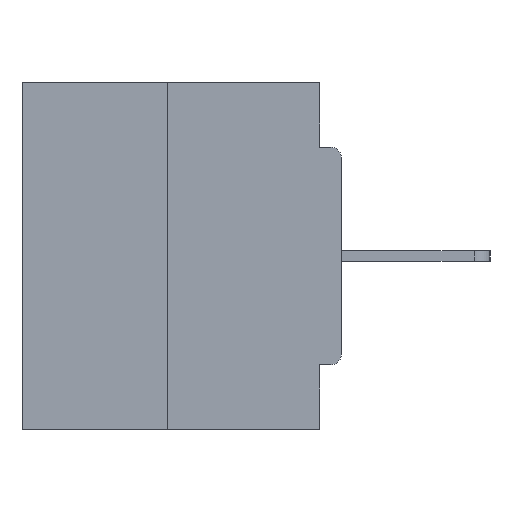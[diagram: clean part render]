
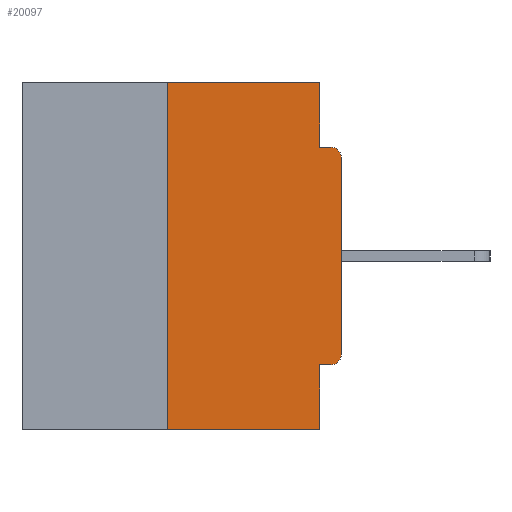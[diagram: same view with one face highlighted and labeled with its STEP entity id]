
A CAD part, left-side view. The second image highlights one B-rep face of the part: STEP entity #20097.
In plain terms, the highlighted planar face has unit normal (-1, 0, 0).
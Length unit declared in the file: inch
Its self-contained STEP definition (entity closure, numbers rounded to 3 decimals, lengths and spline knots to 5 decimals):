
#342 = VECTOR ( 'NONE', #13717, 39.37008 ) ;
#380 = DIRECTION ( 'NONE',  ( 0., 0., 1. ) ) ;
#614 = EDGE_CURVE ( 'NONE', #27230, #2154, #13152, .T. ) ;
#661 = PLANE ( 'NONE',  #5193 ) ;
#723 = AXIS2_PLACEMENT_3D ( 'NONE', #12065, #17318, #14933 ) ;
#757 = ORIENTED_EDGE ( 'NONE', *, *, #18903, .F. ) ;
#862 = ORIENTED_EDGE ( 'NONE', *, *, #25613, .F. ) ;
#1022 = CARTESIAN_POINT ( 'NONE',  ( 0., 0., -0.3915 ) ) ;
#2154 = VERTEX_POINT ( 'NONE', #19680 ) ;
#2256 = DIRECTION ( 'NONE',  ( 0., 0., -1. ) ) ;
#2449 = CARTESIAN_POINT ( 'NONE',  ( 0., 0.46, 0. ) ) ;
#2577 = CARTESIAN_POINT ( 'NONE',  ( 0., 0., 0. ) ) ;
#2992 = DIRECTION ( 'NONE',  ( 0., 0., 1. ) ) ;
#3128 = EDGE_CURVE ( 'NONE', #22360, #9366, #9825, .T. ) ;
#3137 = LINE ( 'NONE', #5524, #28542 ) ;
#3690 = ORIENTED_EDGE ( 'NONE', *, *, #25603, .F. ) ;
#3891 = EDGE_CURVE ( 'NONE', #9366, #13683, #4969, .T. ) ;
#4315 = LINE ( 'NONE', #24075, #11857 ) ;
#4780 = ORIENTED_EDGE ( 'NONE', *, *, #3891, .T. ) ;
#4822 = DIRECTION ( 'NONE',  ( 0., -1., 0. ) ) ;
#4969 = LINE ( 'NONE', #2577, #5308 ) ;
#5193 = AXIS2_PLACEMENT_3D ( 'NONE', #26952, #27274, #24726 ) ;
#5206 = CARTESIAN_POINT ( 'NONE',  ( 0., 0., -0.4065 ) ) ;
#5308 = VECTOR ( 'NONE', #380, 39.37008 ) ;
#5524 = CARTESIAN_POINT ( 'NONE',  ( 0., 0.25, 0. ) ) ;
#6390 = LINE ( 'NONE', #11798, #342 ) ;
#6964 = VERTEX_POINT ( 'NONE', #23285 ) ;
#7230 = VECTOR ( 'NONE', #17772, 39.37008 ) ;
#7241 = CARTESIAN_POINT ( 'NONE',  ( 0., 0., -0.1085 ) ) ;
#8156 = ORIENTED_EDGE ( 'NONE', *, *, #26112, .F. ) ;
#9366 = VERTEX_POINT ( 'NONE', #1022 ) ;
#9825 = CIRCLE ( 'NONE', #25092, 0.015 ) ;
#9902 = EDGE_CURVE ( 'NONE', #17924, #12149, #4315, .T. ) ;
#10376 = CIRCLE ( 'NONE', #723, 0.015 ) ;
#11001 = CARTESIAN_POINT ( 'NONE',  ( 0., 0.015, -0.4065 ) ) ;
#11742 = ORIENTED_EDGE ( 'NONE', *, *, #9902, .F. ) ;
#11798 = CARTESIAN_POINT ( 'NONE',  ( 0., 0.46, -0.5 ) ) ;
#11857 = VECTOR ( 'NONE', #2256, 39.37008 ) ;
#12065 = CARTESIAN_POINT ( 'NONE',  ( 0., 0.015, -0.1085 ) ) ;
#12149 = VERTEX_POINT ( 'NONE', #27022 ) ;
#13152 = LINE ( 'NONE', #30043, #7230 ) ;
#13683 = VERTEX_POINT ( 'NONE', #7241 ) ;
#13717 = DIRECTION ( 'NONE',  ( 0., -1., 0. ) ) ;
#14562 = LINE ( 'NONE', #26670, #14572 ) ;
#14572 = VECTOR ( 'NONE', #4822, 39.37008 ) ;
#14933 = DIRECTION ( 'NONE',  ( 0., 0., -1. ) ) ;
#15132 = DIRECTION ( 'NONE',  ( 0., 0., -1. ) ) ;
#16623 = VECTOR ( 'NONE', #17830, 39.37008 ) ;
#17158 = CARTESIAN_POINT ( 'NONE',  ( 0., 0.25, 0. ) ) ;
#17318 = DIRECTION ( 'NONE',  ( -1., 0., 0. ) ) ;
#17326 = ORIENTED_EDGE ( 'NONE', *, *, #30831, .T. ) ;
#17336 = LINE ( 'NONE', #5206, #18650 ) ;
#17385 = FACE_OUTER_BOUND ( 'NONE', #23309, .T. ) ;
#17772 = DIRECTION ( 'NONE',  ( 0., 0., -1. ) ) ;
#17830 = DIRECTION ( 'NONE',  ( 0., -1., 0. ) ) ;
#17877 = CARTESIAN_POINT ( 'NONE',  ( 0., 0.015, -0.0935 ) ) ;
#17924 = VERTEX_POINT ( 'NONE', #24322 ) ;
#17968 = VERTEX_POINT ( 'NONE', #17158 ) ;
#18650 = VECTOR ( 'NONE', #24355, 39.37008 ) ;
#18903 = EDGE_CURVE ( 'NONE', #6964, #17968, #3137, .T. ) ;
#19680 = CARTESIAN_POINT ( 'NONE',  ( 0., 0.031, -0.5 ) ) ;
#20097 = ADVANCED_FACE ( 'NONE', ( #17385 ), #661, .F. ) ;
#20697 = VERTEX_POINT ( 'NONE', #17877 ) ;
#22360 = VERTEX_POINT ( 'NONE', #11001 ) ;
#22622 = LINE ( 'NONE', #2449, #16623 ) ;
#23068 = DIRECTION ( 'NONE',  ( -1., 0., 0. ) ) ;
#23285 = CARTESIAN_POINT ( 'NONE',  ( 0., 0.25, -0.5 ) ) ;
#23309 = EDGE_LOOP ( 'NONE', ( #862, #757, #30342, #30093, #8156, #28020, #4780, #17326, #3690, #11742 ) ) ;
#24075 = CARTESIAN_POINT ( 'NONE',  ( 0., 0.031, 0. ) ) ;
#24322 = CARTESIAN_POINT ( 'NONE',  ( 0., 0.031, 0. ) ) ;
#24355 = DIRECTION ( 'NONE',  ( 0., 1., 0. ) ) ;
#24726 = DIRECTION ( 'NONE',  ( 0., 0., -1. ) ) ;
#25092 = AXIS2_PLACEMENT_3D ( 'NONE', #27245, #23068, #15132 ) ;
#25525 = CARTESIAN_POINT ( 'NONE',  ( 0., 0.031, -0.4065 ) ) ;
#25603 = EDGE_CURVE ( 'NONE', #12149, #20697, #14562, .T. ) ;
#25613 = EDGE_CURVE ( 'NONE', #17968, #17924, #22622, .T. ) ;
#26112 = EDGE_CURVE ( 'NONE', #22360, #27230, #17336, .T. ) ;
#26670 = CARTESIAN_POINT ( 'NONE',  ( 0., 0., -0.0935 ) ) ;
#26952 = CARTESIAN_POINT ( 'NONE',  ( 0., 0.46, 0. ) ) ;
#27022 = CARTESIAN_POINT ( 'NONE',  ( 0., 0.031, -0.0935 ) ) ;
#27230 = VERTEX_POINT ( 'NONE', #25525 ) ;
#27245 = CARTESIAN_POINT ( 'NONE',  ( 0., 0.015, -0.3915 ) ) ;
#27274 = DIRECTION ( 'NONE',  ( 1., 0., 0. ) ) ;
#27334 = EDGE_CURVE ( 'NONE', #6964, #2154, #6390, .T. ) ;
#28020 = ORIENTED_EDGE ( 'NONE', *, *, #3128, .T. ) ;
#28542 = VECTOR ( 'NONE', #2992, 39.37008 ) ;
#30043 = CARTESIAN_POINT ( 'NONE',  ( 0., 0.031, -0.5 ) ) ;
#30093 = ORIENTED_EDGE ( 'NONE', *, *, #614, .F. ) ;
#30342 = ORIENTED_EDGE ( 'NONE', *, *, #27334, .T. ) ;
#30831 = EDGE_CURVE ( 'NONE', #13683, #20697, #10376, .T. ) ;
